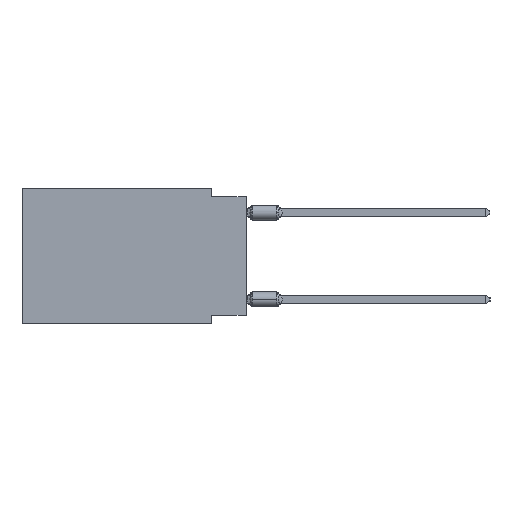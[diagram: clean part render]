
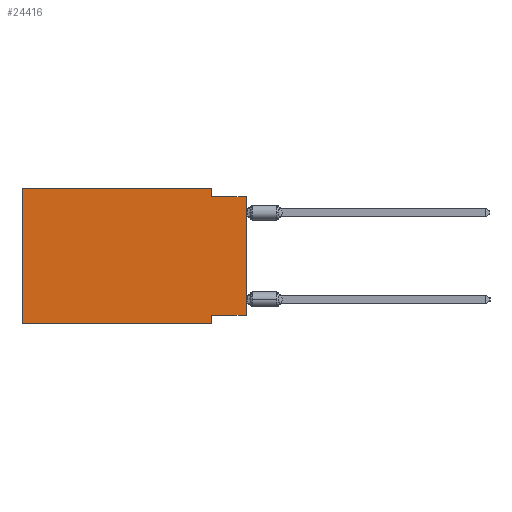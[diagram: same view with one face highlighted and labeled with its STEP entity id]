
A CAD part, left-side view. The second image highlights one B-rep face of the part: STEP entity #24416.
In plain terms, the highlighted planar face has unit normal (-1, 0, 0).
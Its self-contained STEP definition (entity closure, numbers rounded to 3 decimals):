
#783 = VECTOR ( 'NONE', #39337, 1000. ) ;
#1778 = EDGE_CURVE ( 'NONE', #18994, #22427, #46691, .T. ) ;
#2464 = VECTOR ( 'NONE', #28607, 1000. ) ;
#2609 = EDGE_CURVE ( 'NONE', #10392, #18735, #31359, .T. ) ;
#3359 = EDGE_LOOP ( 'NONE', ( #29587, #5929, #43652, #4845, #44419, #40441, #9020, #43063 ) ) ;
#3647 = EDGE_CURVE ( 'NONE', #20460, #18735, #48556, .T. ) ;
#4523 = CARTESIAN_POINT ( 'NONE',  ( 0., 16.383, 0. ) ) ;
#4845 = ORIENTED_EDGE ( 'NONE', *, *, #29682, .F. ) ;
#5411 = CARTESIAN_POINT ( 'NONE',  ( 0., 2.54, -9.271 ) ) ;
#5787 = CARTESIAN_POINT ( 'NONE',  ( 0., 16.383, -9.906 ) ) ;
#5929 = ORIENTED_EDGE ( 'NONE', *, *, #3647, .F. ) ;
#6246 = LINE ( 'NONE', #39038, #783 ) ;
#7275 = EDGE_CURVE ( 'NONE', #10392, #18994, #6246, .T. ) ;
#7772 = CARTESIAN_POINT ( 'NONE',  ( 0., 0., 0. ) ) ;
#9020 = ORIENTED_EDGE ( 'NONE', *, *, #1778, .F. ) ;
#9553 = CARTESIAN_POINT ( 'NONE',  ( 0., 2.54, -9.906 ) ) ;
#10392 = VERTEX_POINT ( 'NONE', #36967 ) ;
#11597 = LINE ( 'NONE', #5787, #16539 ) ;
#12666 = DIRECTION ( 'NONE',  ( 0., 0., 1. ) ) ;
#13872 = LINE ( 'NONE', #32562, #50765 ) ;
#16539 = VECTOR ( 'NONE', #52980, 1000. ) ;
#18528 = CARTESIAN_POINT ( 'NONE',  ( 0., 16.383, 0. ) ) ;
#18735 = VERTEX_POINT ( 'NONE', #25667 ) ;
#18994 = VERTEX_POINT ( 'NONE', #5411 ) ;
#19244 = VECTOR ( 'NONE', #43651, 1000. ) ;
#20460 = VERTEX_POINT ( 'NONE', #40257 ) ;
#20502 = VECTOR ( 'NONE', #27163, 1000. ) ;
#20677 = CARTESIAN_POINT ( 'NONE',  ( 0., 0., -0.635 ) ) ;
#22427 = VERTEX_POINT ( 'NONE', #9553 ) ;
#23123 = AXIS2_PLACEMENT_3D ( 'NONE', #4523, #41920, #47403 ) ;
#24416 = ADVANCED_FACE ( 'NONE', ( #55724 ), #46503, .F. ) ;
#25214 = LINE ( 'NONE', #25515, #50470 ) ;
#25515 = CARTESIAN_POINT ( 'NONE',  ( 0., 2.54, 0. ) ) ;
#25667 = CARTESIAN_POINT ( 'NONE',  ( 0., 0., -0.635 ) ) ;
#27163 = DIRECTION ( 'NONE',  ( 0., -1., 0. ) ) ;
#27213 = CARTESIAN_POINT ( 'NONE',  ( 0., 16.383, -9.906 ) ) ;
#27396 = EDGE_CURVE ( 'NONE', #40520, #34752, #13872, .T. ) ;
#28607 = DIRECTION ( 'NONE',  ( 0., 0., -1. ) ) ;
#29587 = ORIENTED_EDGE ( 'NONE', *, *, #2609, .T. ) ;
#29682 = EDGE_CURVE ( 'NONE', #34752, #35212, #55388, .T. ) ;
#31359 = LINE ( 'NONE', #7772, #41677 ) ;
#32562 = CARTESIAN_POINT ( 'NONE',  ( 0., 16.383, 0. ) ) ;
#34752 = VERTEX_POINT ( 'NONE', #18528 ) ;
#35212 = VERTEX_POINT ( 'NONE', #40857 ) ;
#36967 = CARTESIAN_POINT ( 'NONE',  ( 0., 0., -9.271 ) ) ;
#38108 = CARTESIAN_POINT ( 'NONE',  ( 0., 2.54, -9.906 ) ) ;
#39038 = CARTESIAN_POINT ( 'NONE',  ( 0., 0., -9.271 ) ) ;
#39337 = DIRECTION ( 'NONE',  ( 0., 1., 0. ) ) ;
#40257 = CARTESIAN_POINT ( 'NONE',  ( 0., 2.54, -0.635 ) ) ;
#40441 = ORIENTED_EDGE ( 'NONE', *, *, #55737, .T. ) ;
#40520 = VERTEX_POINT ( 'NONE', #27213 ) ;
#40857 = CARTESIAN_POINT ( 'NONE',  ( 0., 2.54, 0. ) ) ;
#41677 = VECTOR ( 'NONE', #12666, 1000. ) ;
#41920 = DIRECTION ( 'NONE',  ( 1., 0., 0. ) ) ;
#43063 = ORIENTED_EDGE ( 'NONE', *, *, #7275, .F. ) ;
#43651 = DIRECTION ( 'NONE',  ( 0., -1., 0. ) ) ;
#43652 = ORIENTED_EDGE ( 'NONE', *, *, #53631, .F. ) ;
#44419 = ORIENTED_EDGE ( 'NONE', *, *, #27396, .F. ) ;
#46503 = PLANE ( 'NONE',  #23123 ) ;
#46691 = LINE ( 'NONE', #38108, #2464 ) ;
#47403 = DIRECTION ( 'NONE',  ( 0., 0., -1. ) ) ;
#48205 = DIRECTION ( 'NONE',  ( 0., 0., -1. ) ) ;
#48556 = LINE ( 'NONE', #20677, #19244 ) ;
#50470 = VECTOR ( 'NONE', #48205, 1000. ) ;
#50765 = VECTOR ( 'NONE', #51262, 1000. ) ;
#51262 = DIRECTION ( 'NONE',  ( 0., 0., 1. ) ) ;
#52980 = DIRECTION ( 'NONE',  ( 0., -1., 0. ) ) ;
#53631 = EDGE_CURVE ( 'NONE', #35212, #20460, #25214, .T. ) ;
#55388 = LINE ( 'NONE', #60289, #20502 ) ;
#55724 = FACE_OUTER_BOUND ( 'NONE', #3359, .T. ) ;
#55737 = EDGE_CURVE ( 'NONE', #40520, #22427, #11597, .T. ) ;
#60289 = CARTESIAN_POINT ( 'NONE',  ( 0., 16.383, 0. ) ) ;
